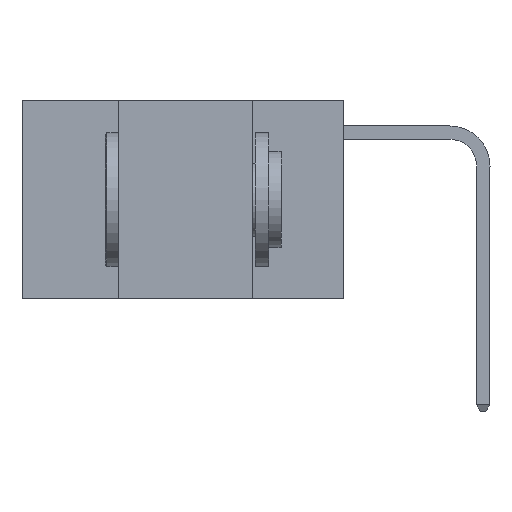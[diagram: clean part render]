
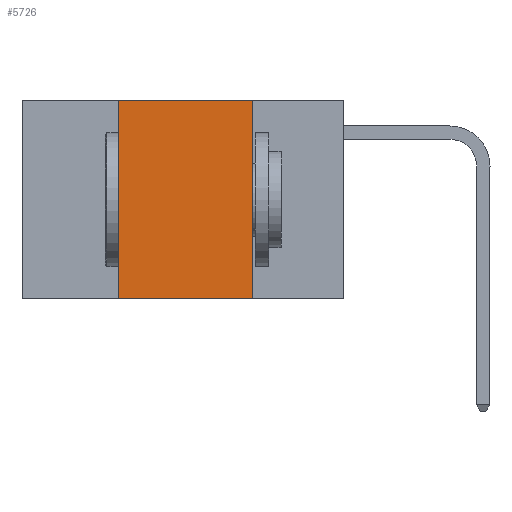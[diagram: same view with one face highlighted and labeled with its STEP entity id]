
A CAD part, left-side view. The second image highlights one B-rep face of the part: STEP entity #5726.
In plain terms, the highlighted planar face has unit normal (-1, 0, 0).
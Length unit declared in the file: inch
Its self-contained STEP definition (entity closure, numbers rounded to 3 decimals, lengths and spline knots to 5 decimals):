
#1351 = EDGE_LOOP ( 'NONE', ( #2542, #6204, #13505, #13930 ) ) ;
#1587 = FACE_OUTER_BOUND ( 'NONE', #1351, .T. ) ;
#1653 = LINE ( 'NONE', #5246, #12247 ) ;
#2542 = ORIENTED_EDGE ( 'NONE', *, *, #2994, .F. ) ;
#2994 = EDGE_CURVE ( 'NONE', #14956, #10458, #9510, .T. ) ;
#3189 = CARTESIAN_POINT ( 'NONE',  ( 0., 0.6, -0.37 ) ) ;
#3647 = DIRECTION ( 'NONE',  ( 0., 0., -1. ) ) ;
#3792 = DIRECTION ( 'NONE',  ( 0., -1., 0. ) ) ;
#3906 = EDGE_CURVE ( 'NONE', #15114, #12379, #1653, .T. ) ;
#4256 = CARTESIAN_POINT ( 'NONE',  ( 0., 0.17, 0. ) ) ;
#4827 = EDGE_CURVE ( 'NONE', #15114, #10458, #13904, .T. ) ;
#5028 = AXIS2_PLACEMENT_3D ( 'NONE', #9327, #16112, #7966 ) ;
#5190 = PLANE ( 'NONE',  #5028 ) ;
#5246 = CARTESIAN_POINT ( 'NONE',  ( 0., 0.42, 0. ) ) ;
#5269 = CARTESIAN_POINT ( 'NONE',  ( 0., 0.42, 0. ) ) ;
#5726 = ADVANCED_FACE ( 'NONE', ( #1587 ), #5190, .F. ) ;
#5729 = CARTESIAN_POINT ( 'NONE',  ( 0., 0.17, -0.37 ) ) ;
#6081 = CARTESIAN_POINT ( 'NONE',  ( 0., 0.17, 0. ) ) ;
#6098 = LINE ( 'NONE', #12055, #13395 ) ;
#6204 = ORIENTED_EDGE ( 'NONE', *, *, #10261, .F. ) ;
#7966 = DIRECTION ( 'NONE',  ( 0., 0., -1. ) ) ;
#9327 = CARTESIAN_POINT ( 'NONE',  ( 0., 0.6, 0. ) ) ;
#9510 = LINE ( 'NONE', #4256, #16671 ) ;
#10261 = EDGE_CURVE ( 'NONE', #12379, #14956, #6098, .T. ) ;
#10458 = VERTEX_POINT ( 'NONE', #5729 ) ;
#10814 = DIRECTION ( 'NONE',  ( 0., 0., 1. ) ) ;
#12055 = CARTESIAN_POINT ( 'NONE',  ( 0., 0.6, 0. ) ) ;
#12247 = VECTOR ( 'NONE', #10814, 39.37008 ) ;
#12379 = VERTEX_POINT ( 'NONE', #5269 ) ;
#13395 = VECTOR ( 'NONE', #3792, 39.37008 ) ;
#13505 = ORIENTED_EDGE ( 'NONE', *, *, #3906, .F. ) ;
#13904 = LINE ( 'NONE', #3189, #17017 ) ;
#13930 = ORIENTED_EDGE ( 'NONE', *, *, #4827, .T. ) ;
#14176 = DIRECTION ( 'NONE',  ( 0., -1., 0. ) ) ;
#14956 = VERTEX_POINT ( 'NONE', #6081 ) ;
#15114 = VERTEX_POINT ( 'NONE', #17290 ) ;
#16112 = DIRECTION ( 'NONE',  ( 1., 0., 0. ) ) ;
#16671 = VECTOR ( 'NONE', #3647, 39.37008 ) ;
#17017 = VECTOR ( 'NONE', #14176, 39.37008 ) ;
#17290 = CARTESIAN_POINT ( 'NONE',  ( 0., 0.42, -0.37 ) ) ;
